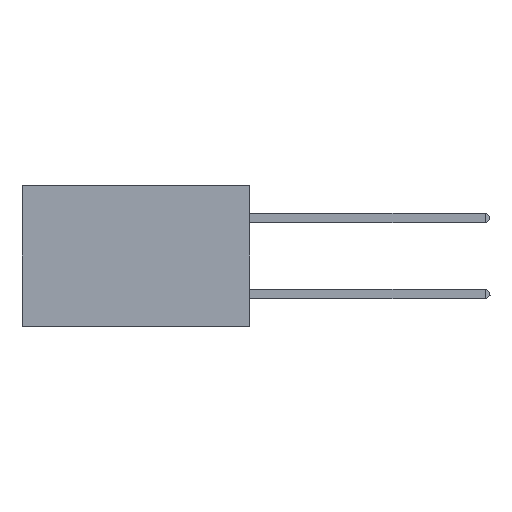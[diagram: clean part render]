
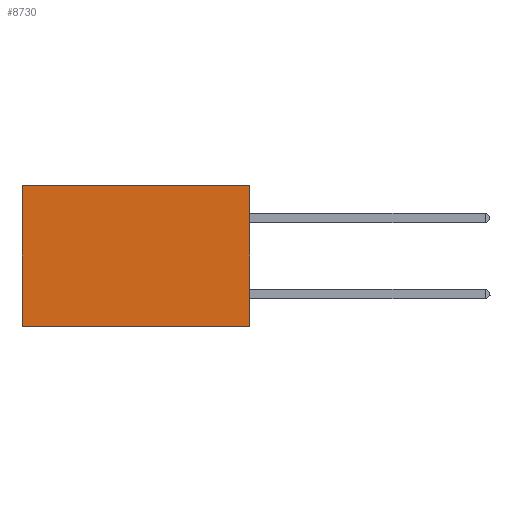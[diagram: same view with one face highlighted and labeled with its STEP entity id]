
A CAD part, left-side view. The second image highlights one B-rep face of the part: STEP entity #8730.
In plain terms, the highlighted planar face has unit normal (-1, 0, 0).
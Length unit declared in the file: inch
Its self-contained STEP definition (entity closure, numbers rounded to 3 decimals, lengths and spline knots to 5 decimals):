
#270 = VERTEX_POINT ( 'NONE', #5309 ) ;
#2925 = DIRECTION ( 'NONE',  ( 0., 0., -1. ) ) ;
#3097 = DIRECTION ( 'NONE',  ( 1., 0., 0. ) ) ;
#3368 = VERTEX_POINT ( 'NONE', #22686 ) ;
#3999 = DIRECTION ( 'NONE',  ( 0., 1., 0. ) ) ;
#4060 = EDGE_CURVE ( 'NONE', #3368, #14331, #25127, .T. ) ;
#4436 = AXIS2_PLACEMENT_3D ( 'NONE', #18902, #3097, #17001 ) ;
#4567 = VECTOR ( 'NONE', #2925, 39.37008 ) ;
#5309 = CARTESIAN_POINT ( 'NONE',  ( 0.2875, 0.6, 0. ) ) ;
#5743 = LINE ( 'NONE', #21656, #13078 ) ;
#7045 = VERTEX_POINT ( 'NONE', #19187 ) ;
#7502 = EDGE_CURVE ( 'NONE', #7045, #3368, #18745, .T. ) ;
#7523 = ORIENTED_EDGE ( 'NONE', *, *, #4060, .F. ) ;
#8249 = ORIENTED_EDGE ( 'NONE', *, *, #7502, .F. ) ;
#8392 = ORIENTED_EDGE ( 'NONE', *, *, #21670, .T. ) ;
#8730 = ADVANCED_FACE ( 'NONE', ( #14677 ), #24595, .F. ) ;
#9265 = VECTOR ( 'NONE', #20511, 39.37008 ) ;
#9652 = EDGE_CURVE ( 'NONE', #7045, #270, #5743, .T. ) ;
#10417 = ORIENTED_EDGE ( 'NONE', *, *, #9652, .T. ) ;
#13078 = VECTOR ( 'NONE', #3999, 39.37008 ) ;
#14331 = VERTEX_POINT ( 'NONE', #16299 ) ;
#14671 = DIRECTION ( 'NONE',  ( 0., 0., -1. ) ) ;
#14677 = FACE_OUTER_BOUND ( 'NONE', #19002, .T. ) ;
#15371 = VECTOR ( 'NONE', #14671, 39.37008 ) ;
#15431 = CARTESIAN_POINT ( 'NONE',  ( 0.2875, 0., -0.37 ) ) ;
#16299 = CARTESIAN_POINT ( 'NONE',  ( 0.2875, 0.6, -0.37 ) ) ;
#16743 = CARTESIAN_POINT ( 'NONE',  ( 0.2875, 0., 0. ) ) ;
#17001 = DIRECTION ( 'NONE',  ( 0., 0., -1. ) ) ;
#18745 = LINE ( 'NONE', #16743, #4567 ) ;
#18902 = CARTESIAN_POINT ( 'NONE',  ( 0.2875, 0., 0. ) ) ;
#19002 = EDGE_LOOP ( 'NONE', ( #8392, #7523, #8249, #10417 ) ) ;
#19187 = CARTESIAN_POINT ( 'NONE',  ( 0.2875, 0., 0. ) ) ;
#20511 = DIRECTION ( 'NONE',  ( 0., 1., 0. ) ) ;
#21656 = CARTESIAN_POINT ( 'NONE',  ( 0.2875, 0., 0. ) ) ;
#21670 = EDGE_CURVE ( 'NONE', #270, #14331, #21908, .T. ) ;
#21908 = LINE ( 'NONE', #22584, #15371 ) ;
#22584 = CARTESIAN_POINT ( 'NONE',  ( 0.2875, 0.6, 0. ) ) ;
#22686 = CARTESIAN_POINT ( 'NONE',  ( 0.2875, 0., -0.37 ) ) ;
#24595 = PLANE ( 'NONE',  #4436 ) ;
#25127 = LINE ( 'NONE', #15431, #9265 ) ;
